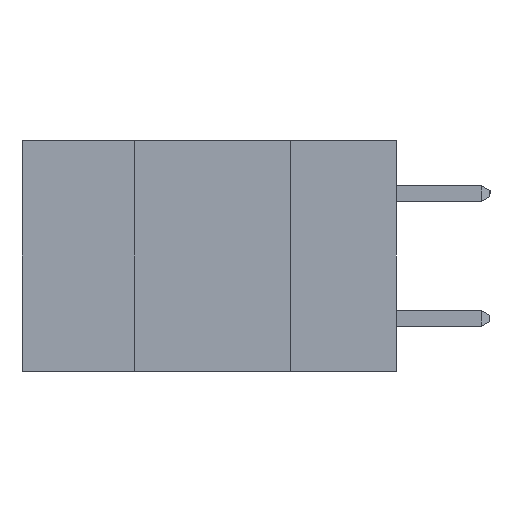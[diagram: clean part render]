
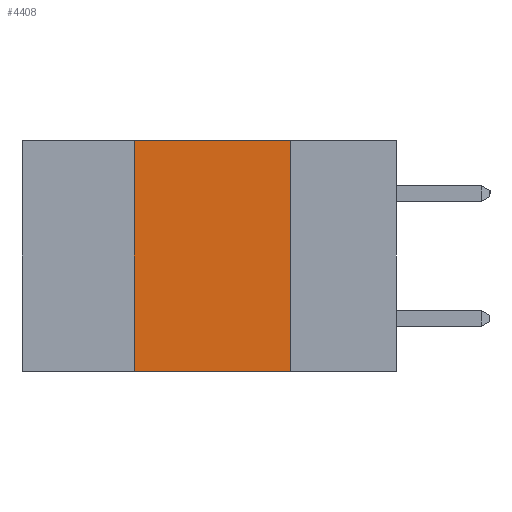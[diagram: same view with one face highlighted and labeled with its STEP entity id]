
A CAD part, left-side view. The second image highlights one B-rep face of the part: STEP entity #4408.
In plain terms, the highlighted planar face has unit normal (-1, 0, 0).
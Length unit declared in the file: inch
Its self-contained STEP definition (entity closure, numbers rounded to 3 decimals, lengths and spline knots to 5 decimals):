
#431 = CARTESIAN_POINT ( 'NONE',  ( 0., 0.6, 0. ) ) ;
#460 = CARTESIAN_POINT ( 'NONE',  ( 0., 0.6, -0.37 ) ) ;
#461 = ORIENTED_EDGE ( 'NONE', *, *, #527, .F. ) ;
#527 = EDGE_CURVE ( 'NONE', #8238, #3366, #1320, .T. ) ;
#1070 = VECTOR ( 'NONE', #2022, 39.37008 ) ;
#1077 = LINE ( 'NONE', #2905, #1070 ) ;
#1320 = LINE ( 'NONE', #8774, #8099 ) ;
#1351 = VECTOR ( 'NONE', #6773, 39.37008 ) ;
#2022 = DIRECTION ( 'NONE',  ( 0., 0., 1. ) ) ;
#2842 = VECTOR ( 'NONE', #3779, 39.37008 ) ;
#2884 = EDGE_CURVE ( 'NONE', #6574, #8238, #4356, .T. ) ;
#2905 = CARTESIAN_POINT ( 'NONE',  ( 0., 0.42, -0.37 ) ) ;
#3282 = CARTESIAN_POINT ( 'NONE',  ( 0., 0.17, 0. ) ) ;
#3366 = VERTEX_POINT ( 'NONE', #5251 ) ;
#3398 = CARTESIAN_POINT ( 'NONE',  ( 0., 0.42, -0.37 ) ) ;
#3779 = DIRECTION ( 'NONE',  ( 0., -1., 0. ) ) ;
#3792 = DIRECTION ( 'NONE',  ( 1., 0., 0. ) ) ;
#4356 = LINE ( 'NONE', #5018, #1351 ) ;
#4408 = ADVANCED_FACE ( 'NONE', ( #7979 ), #6372, .F. ) ;
#5018 = CARTESIAN_POINT ( 'NONE',  ( 0., 0.6, 0. ) ) ;
#5243 = EDGE_LOOP ( 'NONE', ( #461, #5582, #9820, #6640 ) ) ;
#5251 = CARTESIAN_POINT ( 'NONE',  ( 0., 0.17, -0.37 ) ) ;
#5582 = ORIENTED_EDGE ( 'NONE', *, *, #2884, .F. ) ;
#6372 = PLANE ( 'NONE',  #7159 ) ;
#6574 = VERTEX_POINT ( 'NONE', #10100 ) ;
#6640 = ORIENTED_EDGE ( 'NONE', *, *, #8576, .T. ) ;
#6773 = DIRECTION ( 'NONE',  ( 0., -1., 0. ) ) ;
#7128 = LINE ( 'NONE', #460, #2842 ) ;
#7143 = DIRECTION ( 'NONE',  ( 0., 0., -1. ) ) ;
#7159 = AXIS2_PLACEMENT_3D ( 'NONE', #431, #3792, #7143 ) ;
#7979 = FACE_OUTER_BOUND ( 'NONE', #5243, .T. ) ;
#8099 = VECTOR ( 'NONE', #10397, 39.37008 ) ;
#8238 = VERTEX_POINT ( 'NONE', #3282 ) ;
#8288 = VERTEX_POINT ( 'NONE', #3398 ) ;
#8576 = EDGE_CURVE ( 'NONE', #8288, #3366, #7128, .T. ) ;
#8774 = CARTESIAN_POINT ( 'NONE',  ( 0., 0.17, -0.37 ) ) ;
#9259 = EDGE_CURVE ( 'NONE', #8288, #6574, #1077, .T. ) ;
#9820 = ORIENTED_EDGE ( 'NONE', *, *, #9259, .F. ) ;
#10100 = CARTESIAN_POINT ( 'NONE',  ( 0., 0.42, 0. ) ) ;
#10397 = DIRECTION ( 'NONE',  ( 0., 0., -1. ) ) ;
